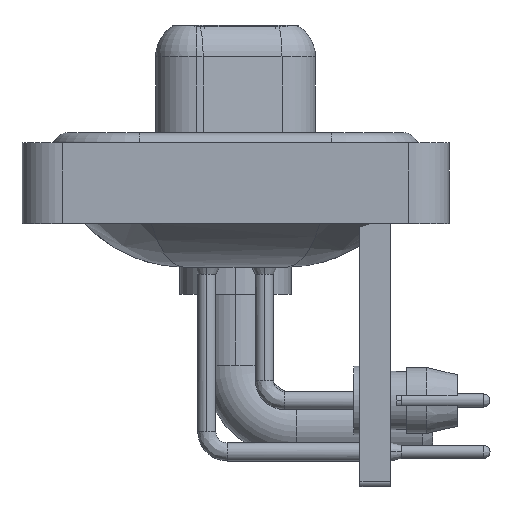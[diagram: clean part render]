
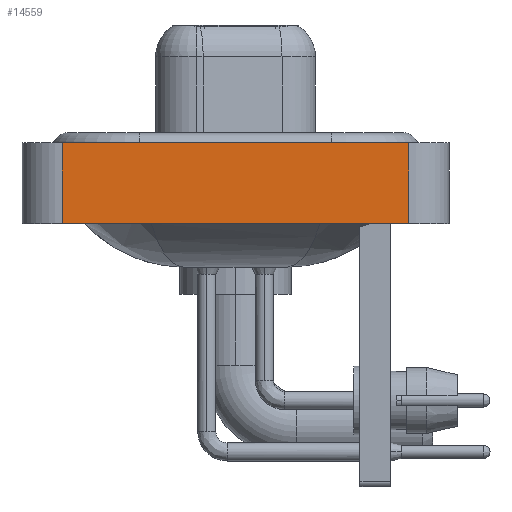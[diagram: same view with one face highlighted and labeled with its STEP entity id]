
A CAD part, left-side view. The second image highlights one B-rep face of the part: STEP entity #14559.
In plain terms, the highlighted planar face has unit normal (-1, 0, 0).
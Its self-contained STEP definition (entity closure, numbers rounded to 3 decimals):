
#617 = ORIENTED_EDGE ( 'NONE', *, *, #13747, .F. ) ;
#1599 = VERTEX_POINT ( 'NONE', #6583 ) ;
#1728 = DIRECTION ( 'NONE',  ( 0., 0., 1. ) ) ;
#1928 = LINE ( 'NONE', #8828, #21369 ) ;
#2394 = CARTESIAN_POINT ( 'NONE',  ( -7.25, 8.55, -3.6 ) ) ;
#2485 = ORIENTED_EDGE ( 'NONE', *, *, #17442, .T. ) ;
#3093 = VERTEX_POINT ( 'NONE', #3316 ) ;
#3291 = EDGE_CURVE ( 'NONE', #7203, #1599, #16176, .T. ) ;
#3316 = CARTESIAN_POINT ( 'NONE',  ( -7.25, -8.55, 0.4 ) ) ;
#3408 = CARTESIAN_POINT ( 'NONE',  ( -7.25, -8.55, -3.6 ) ) ;
#3576 = EDGE_CURVE ( 'NONE', #20439, #3093, #1928, .T. ) ;
#4520 = VECTOR ( 'NONE', #15768, 1000. ) ;
#4545 = EDGE_LOOP ( 'NONE', ( #16921, #617, #15002, #2485 ) ) ;
#5010 = CARTESIAN_POINT ( 'NONE',  ( -7.25, -8.55, -3.6 ) ) ;
#5571 = DIRECTION ( 'NONE',  ( 0., 0., 1. ) ) ;
#6583 = CARTESIAN_POINT ( 'NONE',  ( -7.25, 8.55, 0.4 ) ) ;
#6966 = LINE ( 'NONE', #8893, #4520 ) ;
#7203 = VERTEX_POINT ( 'NONE', #17269 ) ;
#8828 = CARTESIAN_POINT ( 'NONE',  ( -7.25, -8.55, -3.6 ) ) ;
#8893 = CARTESIAN_POINT ( 'NONE',  ( -7.25, -8.55, -3.6 ) ) ;
#10327 = PLANE ( 'NONE',  #19368 ) ;
#11765 = CARTESIAN_POINT ( 'NONE',  ( -7.25, -8.55, 0.4 ) ) ;
#12020 = FACE_OUTER_BOUND ( 'NONE', #4545, .T. ) ;
#12653 = DIRECTION ( 'NONE',  ( 0., 0., 1. ) ) ;
#13747 = EDGE_CURVE ( 'NONE', #1599, #3093, #13791, .T. ) ;
#13791 = LINE ( 'NONE', #11765, #15068 ) ;
#14559 = ADVANCED_FACE ( 'NONE', ( #12020 ), #10327, .T. ) ;
#15002 = ORIENTED_EDGE ( 'NONE', *, *, #3291, .F. ) ;
#15068 = VECTOR ( 'NONE', #20669, 1000. ) ;
#15768 = DIRECTION ( 'NONE',  ( 0., -1., 0. ) ) ;
#16176 = LINE ( 'NONE', #2394, #19246 ) ;
#16921 = ORIENTED_EDGE ( 'NONE', *, *, #3576, .T. ) ;
#17269 = CARTESIAN_POINT ( 'NONE',  ( -7.25, 8.55, -3.6 ) ) ;
#17442 = EDGE_CURVE ( 'NONE', #7203, #20439, #6966, .T. ) ;
#18548 = DIRECTION ( 'NONE',  ( -1., 0., 0. ) ) ;
#19246 = VECTOR ( 'NONE', #5571, 1000. ) ;
#19368 = AXIS2_PLACEMENT_3D ( 'NONE', #5010, #18548, #1728 ) ;
#20439 = VERTEX_POINT ( 'NONE', #3408 ) ;
#20669 = DIRECTION ( 'NONE',  ( 0., -1., 0. ) ) ;
#21369 = VECTOR ( 'NONE', #12653, 1000. ) ;
